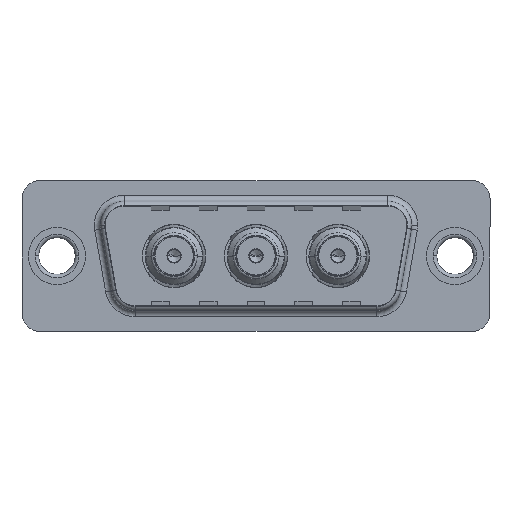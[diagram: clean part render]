
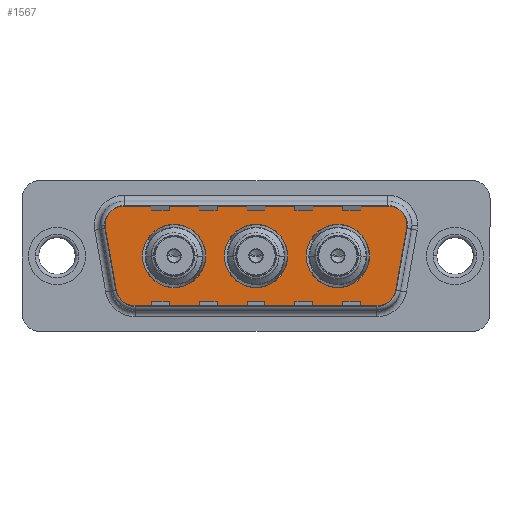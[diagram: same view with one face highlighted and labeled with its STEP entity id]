
A CAD part, top view. The second image highlights one B-rep face of the part: STEP entity #1567.
In plain terms, the highlighted planar face has unit normal (0, 0, 1).
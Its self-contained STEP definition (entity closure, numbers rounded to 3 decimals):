
#30 = VERTEX_POINT ( 'NONE', #7511 ) ;
#43 = ORIENTED_EDGE ( 'NONE', *, *, #1858, .F. ) ;
#273 = EDGE_CURVE ( 'NONE', #2866, #1707, #13498, .T. ) ;
#298 = CARTESIAN_POINT ( 'NONE',  ( 6.434, -4.9, 0. ) ) ;
#334 = DIRECTION ( 'NONE',  ( 1., 0., 0. ) ) ;
#357 = VECTOR ( 'NONE', #11406, 1000. ) ;
#444 = DIRECTION ( 'NONE',  ( 0., 0., 1. ) ) ;
#465 = EDGE_CURVE ( 'NONE', #3708, #9825, #10453, .T. ) ;
#659 = EDGE_LOOP ( 'NONE', ( #7530, #1108 ) ) ;
#781 = CIRCLE ( 'NONE', #7784, 2.65 ) ;
#974 = CARTESIAN_POINT ( 'NONE',  ( 7.15, 0., 0. ) ) ;
#992 = DIRECTION ( 'NONE',  ( 0., 0., 1. ) ) ;
#1061 = CIRCLE ( 'NONE', #8474, 2.65 ) ;
#1073 = CARTESIAN_POINT ( 'NONE',  ( 6.434, -4.9, 0. ) ) ;
#1108 = ORIENTED_EDGE ( 'NONE', *, *, #11670, .F. ) ;
#1389 = CARTESIAN_POINT ( 'NONE',  ( 26.15, 0., 0. ) ) ;
#1401 = VERTEX_POINT ( 'NONE', #10997 ) ;
#1510 = EDGE_LOOP ( 'NONE', ( #43, #10780 ) ) ;
#1511 = ORIENTED_EDGE ( 'NONE', *, *, #9304, .F. ) ;
#1567 = ADVANCED_FACE ( 'NONE', ( #1889, #7557, #10769, #12939 ), #10215, .T. ) ;
#1582 = EDGE_CURVE ( 'NONE', #12134, #3708, #4168, .T. ) ;
#1586 = AXIS2_PLACEMENT_3D ( 'NONE', #8864, #13084, #8939 ) ;
#1603 = LINE ( 'NONE', #2721, #4556 ) ;
#1707 = VERTEX_POINT ( 'NONE', #1073 ) ;
#1709 = CIRCLE ( 'NONE', #7836, 2.65 ) ;
#1764 = DIRECTION ( 'NONE',  ( 1., 0., 0. ) ) ;
#1840 = CARTESIAN_POINT ( 'NONE',  ( 4.464, -3.247, 0. ) ) ;
#1858 = EDGE_CURVE ( 'NONE', #1401, #13019, #1709, .T. ) ;
#1889 = FACE_BOUND ( 'NONE', #12253, .T. ) ;
#2721 = CARTESIAN_POINT ( 'NONE',  ( 3.441, 2.553, 0. ) ) ;
#2734 = DIRECTION ( 'NONE',  ( 0., 0., 1. ) ) ;
#2866 = VERTEX_POINT ( 'NONE', #1840 ) ;
#2982 = CIRCLE ( 'NONE', #1586, 2. ) ;
#3031 = ORIENTED_EDGE ( 'NONE', *, *, #6866, .T. ) ;
#3174 = DIRECTION ( 'NONE',  ( 0., 0., 1. ) ) ;
#3235 = VERTEX_POINT ( 'NONE', #7990 ) ;
#3296 = CIRCLE ( 'NONE', #8135, 2. ) ;
#3417 = LINE ( 'NONE', #5769, #11913 ) ;
#3546 = EDGE_CURVE ( 'NONE', #13875, #30, #3417, .T. ) ;
#3548 = EDGE_LOOP ( 'NONE', ( #8962, #6466, #14010, #3031, #11673, #10510, #9299, #8507, #7067 ) ) ;
#3643 = LINE ( 'NONE', #298, #357 ) ;
#3708 = VERTEX_POINT ( 'NONE', #7798 ) ;
#3719 = CARTESIAN_POINT ( 'NONE',  ( 6.434, -2.9, 0. ) ) ;
#3730 = AXIS2_PLACEMENT_3D ( 'NONE', #12702, #5366, #4515 ) ;
#3826 = VERTEX_POINT ( 'NONE', #7627 ) ;
#3881 = DIRECTION ( 'NONE',  ( 0.174, -0.985, 0. ) ) ;
#3920 = CIRCLE ( 'NONE', #4644, 2. ) ;
#4168 = LINE ( 'NONE', #8188, #12626 ) ;
#4515 = DIRECTION ( 'NONE',  ( 1., 0., 0. ) ) ;
#4556 = VECTOR ( 'NONE', #3881, 1000. ) ;
#4644 = AXIS2_PLACEMENT_3D ( 'NONE', #14088, #9126, #8935 ) ;
#4934 = AXIS2_PLACEMENT_3D ( 'NONE', #3719, #8661, #11221 ) ;
#5246 = VERTEX_POINT ( 'NONE', #1389 ) ;
#5366 = DIRECTION ( 'NONE',  ( 0., 0., 1. ) ) ;
#5580 = DIRECTION ( 'NONE',  ( -1., 0., 0. ) ) ;
#5769 = CARTESIAN_POINT ( 'NONE',  ( 5.411, 4.9, 0. ) ) ;
#5898 = CIRCLE ( 'NONE', #6829, 2.65 ) ;
#6177 = AXIS2_PLACEMENT_3D ( 'NONE', #9552, #9228, #12503 ) ;
#6200 = CARTESIAN_POINT ( 'NONE',  ( 29.889, 2.9, 0. ) ) ;
#6364 = EDGE_CURVE ( 'NONE', #5246, #3826, #8003, .T. ) ;
#6466 = ORIENTED_EDGE ( 'NONE', *, *, #1582, .T. ) ;
#6692 = CARTESIAN_POINT ( 'NONE',  ( 19.3, 0., 0. ) ) ;
#6829 = AXIS2_PLACEMENT_3D ( 'NONE', #7161, #444, #8258 ) ;
#6866 = EDGE_CURVE ( 'NONE', #9825, #13875, #3920, .T. ) ;
#6914 = DIRECTION ( 'NONE',  ( 0.174, 0.985, 0. ) ) ;
#7044 = DIRECTION ( 'NONE',  ( 0., 0., 1. ) ) ;
#7067 = ORIENTED_EDGE ( 'NONE', *, *, #10773, .T. ) ;
#7161 = CARTESIAN_POINT ( 'NONE',  ( 16.65, 0., 0. ) ) ;
#7511 = CARTESIAN_POINT ( 'NONE',  ( 5.411, 4.9, 0. ) ) ;
#7530 = ORIENTED_EDGE ( 'NONE', *, *, #6364, .F. ) ;
#7533 = EDGE_CURVE ( 'NONE', #10135, #12134, #2982, .T. ) ;
#7557 = FACE_BOUND ( 'NONE', #659, .T. ) ;
#7627 = CARTESIAN_POINT ( 'NONE',  ( 20.85, 0., 0. ) ) ;
#7731 = CARTESIAN_POINT ( 'NONE',  ( 16.65, 0., 0. ) ) ;
#7784 = AXIS2_PLACEMENT_3D ( 'NONE', #13531, #7044, #334 ) ;
#7798 = CARTESIAN_POINT ( 'NONE',  ( 29.859, 2.553, 0. ) ) ;
#7836 = AXIS2_PLACEMENT_3D ( 'NONE', #8696, #9253, #11785 ) ;
#7926 = ORIENTED_EDGE ( 'NONE', *, *, #10828, .F. ) ;
#7990 = CARTESIAN_POINT ( 'NONE',  ( 14., 0., 0. ) ) ;
#8003 = CIRCLE ( 'NONE', #3730, 2.65 ) ;
#8135 = AXIS2_PLACEMENT_3D ( 'NONE', #9410, #2734, #10533 ) ;
#8188 = CARTESIAN_POINT ( 'NONE',  ( 29.859, 2.553, 0. ) ) ;
#8258 = DIRECTION ( 'NONE',  ( 1., 0., 0. ) ) ;
#8354 = CARTESIAN_POINT ( 'NONE',  ( 27.889, 4.9, 0. ) ) ;
#8474 = AXIS2_PLACEMENT_3D ( 'NONE', #7731, #992, #8816 ) ;
#8507 = ORIENTED_EDGE ( 'NONE', *, *, #273, .T. ) ;
#8661 = DIRECTION ( 'NONE',  ( 0., 0., 1. ) ) ;
#8696 = CARTESIAN_POINT ( 'NONE',  ( 9.8, 0., 0. ) ) ;
#8816 = DIRECTION ( 'NONE',  ( 1., 0., 0. ) ) ;
#8864 = CARTESIAN_POINT ( 'NONE',  ( 26.866, -2.9, 0. ) ) ;
#8935 = DIRECTION ( 'NONE',  ( -1., 0., 0. ) ) ;
#8939 = DIRECTION ( 'NONE',  ( 1., 0., 0. ) ) ;
#8962 = ORIENTED_EDGE ( 'NONE', *, *, #7533, .T. ) ;
#9126 = DIRECTION ( 'NONE',  ( 0., 0., 1. ) ) ;
#9228 = DIRECTION ( 'NONE',  ( 0., 0., 1. ) ) ;
#9253 = DIRECTION ( 'NONE',  ( 0., 0., 1. ) ) ;
#9299 = ORIENTED_EDGE ( 'NONE', *, *, #13870, .T. ) ;
#9304 = EDGE_CURVE ( 'NONE', #11737, #3235, #1061, .T. ) ;
#9410 = CARTESIAN_POINT ( 'NONE',  ( 5.411, 2.9, 0. ) ) ;
#9552 = CARTESIAN_POINT ( 'NONE',  ( 27.889, 2.9, 0. ) ) ;
#9825 = VERTEX_POINT ( 'NONE', #6200 ) ;
#9845 = CARTESIAN_POINT ( 'NONE',  ( 23.5, 0., 0. ) ) ;
#10135 = VERTEX_POINT ( 'NONE', #13418 ) ;
#10215 = PLANE ( 'NONE',  #13138 ) ;
#10230 = CARTESIAN_POINT ( 'NONE',  ( 26.866, -2.9, 0. ) ) ;
#10255 = EDGE_CURVE ( 'NONE', #30, #11703, #3296, .T. ) ;
#10453 = CIRCLE ( 'NONE', #6177, 2. ) ;
#10510 = ORIENTED_EDGE ( 'NONE', *, *, #10255, .T. ) ;
#10533 = DIRECTION ( 'NONE',  ( 1., 0., 0. ) ) ;
#10610 = CARTESIAN_POINT ( 'NONE',  ( 28.836, -3.247, 0. ) ) ;
#10769 = FACE_BOUND ( 'NONE', #1510, .T. ) ;
#10773 = EDGE_CURVE ( 'NONE', #1707, #10135, #3643, .T. ) ;
#10780 = ORIENTED_EDGE ( 'NONE', *, *, #11388, .F. ) ;
#10828 = EDGE_CURVE ( 'NONE', #3235, #11737, #5898, .T. ) ;
#10981 = DIRECTION ( 'NONE',  ( 1., 0., 0. ) ) ;
#10997 = CARTESIAN_POINT ( 'NONE',  ( 12.45, 0., 0. ) ) ;
#11030 = CARTESIAN_POINT ( 'NONE',  ( 3.441, 2.553, 0. ) ) ;
#11221 = DIRECTION ( 'NONE',  ( -1., 0., 0. ) ) ;
#11388 = EDGE_CURVE ( 'NONE', #13019, #1401, #781, .T. ) ;
#11406 = DIRECTION ( 'NONE',  ( 1., 0., 0. ) ) ;
#11670 = EDGE_CURVE ( 'NONE', #3826, #5246, #12037, .T. ) ;
#11673 = ORIENTED_EDGE ( 'NONE', *, *, #3546, .T. ) ;
#11703 = VERTEX_POINT ( 'NONE', #11030 ) ;
#11737 = VERTEX_POINT ( 'NONE', #6692 ) ;
#11785 = DIRECTION ( 'NONE',  ( 1., 0., 0. ) ) ;
#11913 = VECTOR ( 'NONE', #5580, 1000. ) ;
#11969 = DIRECTION ( 'NONE',  ( 0., 0., 1. ) ) ;
#12037 = CIRCLE ( 'NONE', #12594, 2.65 ) ;
#12134 = VERTEX_POINT ( 'NONE', #10610 ) ;
#12253 = EDGE_LOOP ( 'NONE', ( #1511, #7926 ) ) ;
#12503 = DIRECTION ( 'NONE',  ( -1., 0., 0. ) ) ;
#12594 = AXIS2_PLACEMENT_3D ( 'NONE', #9845, #3174, #10981 ) ;
#12626 = VECTOR ( 'NONE', #6914, 1000. ) ;
#12702 = CARTESIAN_POINT ( 'NONE',  ( 23.5, 0., 0. ) ) ;
#12939 = FACE_OUTER_BOUND ( 'NONE', #3548, .T. ) ;
#13019 = VERTEX_POINT ( 'NONE', #974 ) ;
#13084 = DIRECTION ( 'NONE',  ( 0., 0., 1. ) ) ;
#13138 = AXIS2_PLACEMENT_3D ( 'NONE', #10230, #11969, #1764 ) ;
#13418 = CARTESIAN_POINT ( 'NONE',  ( 26.866, -4.9, 0. ) ) ;
#13498 = CIRCLE ( 'NONE', #4934, 2. ) ;
#13531 = CARTESIAN_POINT ( 'NONE',  ( 9.8, 0., 0. ) ) ;
#13870 = EDGE_CURVE ( 'NONE', #11703, #2866, #1603, .T. ) ;
#13875 = VERTEX_POINT ( 'NONE', #8354 ) ;
#14010 = ORIENTED_EDGE ( 'NONE', *, *, #465, .T. ) ;
#14088 = CARTESIAN_POINT ( 'NONE',  ( 27.889, 2.9, 0. ) ) ;
